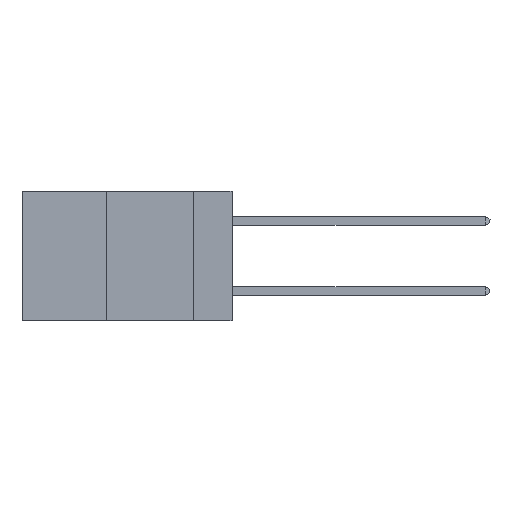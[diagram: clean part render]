
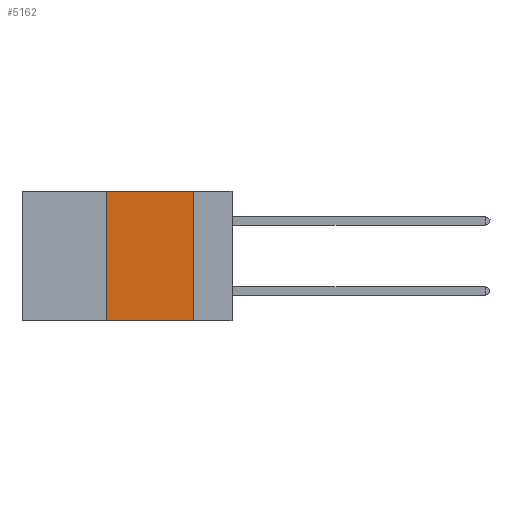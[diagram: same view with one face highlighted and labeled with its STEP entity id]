
A CAD part, left-side view. The second image highlights one B-rep face of the part: STEP entity #5162.
In plain terms, the highlighted planar face has unit normal (-1, 0, 0).
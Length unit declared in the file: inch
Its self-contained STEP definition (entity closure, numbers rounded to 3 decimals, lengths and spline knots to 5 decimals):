
#997 = VECTOR ( 'NONE', #24201, 39.37008 ) ;
#1238 = CARTESIAN_POINT ( 'NONE',  ( 0., 0.11, -0.37 ) ) ;
#1601 = DIRECTION ( 'NONE',  ( 0., 0., 1. ) ) ;
#1839 = VECTOR ( 'NONE', #22139, 39.37008 ) ;
#2355 = CARTESIAN_POINT ( 'NONE',  ( 0., 0.6, 0. ) ) ;
#2470 = DIRECTION ( 'NONE',  ( 0., 0., -1. ) ) ;
#3576 = VECTOR ( 'NONE', #1601, 39.37008 ) ;
#4209 = EDGE_CURVE ( 'NONE', #4793, #21453, #29872, .T. ) ;
#4691 = ORIENTED_EDGE ( 'NONE', *, *, #4209, .F. ) ;
#4793 = VERTEX_POINT ( 'NONE', #26165 ) ;
#5162 = ADVANCED_FACE ( 'NONE', ( #24069 ), #16424, .F. ) ;
#5223 = VERTEX_POINT ( 'NONE', #1238 ) ;
#5289 = DIRECTION ( 'NONE',  ( 1., 0., 0. ) ) ;
#7216 = CARTESIAN_POINT ( 'NONE',  ( 0., 0.36, 0. ) ) ;
#8026 = EDGE_CURVE ( 'NONE', #18305, #5223, #17002, .T. ) ;
#8280 = EDGE_CURVE ( 'NONE', #21453, #18305, #16621, .T. ) ;
#9286 = CARTESIAN_POINT ( 'NONE',  ( 0., 0.11, 0. ) ) ;
#11228 = CARTESIAN_POINT ( 'NONE',  ( 0., 0.36, 0. ) ) ;
#12200 = ORIENTED_EDGE ( 'NONE', *, *, #8280, .F. ) ;
#15352 = EDGE_LOOP ( 'NONE', ( #23579, #12200, #4691, #17567 ) ) ;
#16424 = PLANE ( 'NONE',  #17516 ) ;
#16621 = LINE ( 'NONE', #2355, #29938 ) ;
#17002 = LINE ( 'NONE', #9286, #997 ) ;
#17400 = LINE ( 'NONE', #29681, #1839 ) ;
#17516 = AXIS2_PLACEMENT_3D ( 'NONE', #19183, #5289, #2470 ) ;
#17567 = ORIENTED_EDGE ( 'NONE', *, *, #18850, .T. ) ;
#18305 = VERTEX_POINT ( 'NONE', #19840 ) ;
#18850 = EDGE_CURVE ( 'NONE', #4793, #5223, #17400, .T. ) ;
#19183 = CARTESIAN_POINT ( 'NONE',  ( 0., 0.6, 0. ) ) ;
#19840 = CARTESIAN_POINT ( 'NONE',  ( 0., 0.11, 0. ) ) ;
#21453 = VERTEX_POINT ( 'NONE', #7216 ) ;
#21846 = DIRECTION ( 'NONE',  ( 0., -1., 0. ) ) ;
#22139 = DIRECTION ( 'NONE',  ( 0., -1., 0. ) ) ;
#23579 = ORIENTED_EDGE ( 'NONE', *, *, #8026, .F. ) ;
#24069 = FACE_OUTER_BOUND ( 'NONE', #15352, .T. ) ;
#24201 = DIRECTION ( 'NONE',  ( 0., 0., -1. ) ) ;
#26165 = CARTESIAN_POINT ( 'NONE',  ( 0., 0.36, -0.37 ) ) ;
#29681 = CARTESIAN_POINT ( 'NONE',  ( 0., 0.6, -0.37 ) ) ;
#29872 = LINE ( 'NONE', #11228, #3576 ) ;
#29938 = VECTOR ( 'NONE', #21846, 39.37008 ) ;
